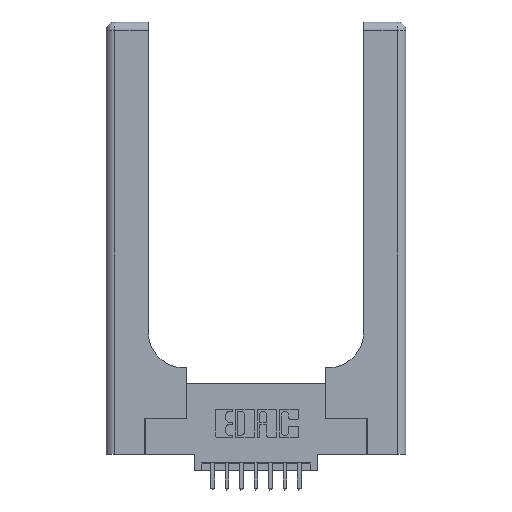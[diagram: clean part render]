
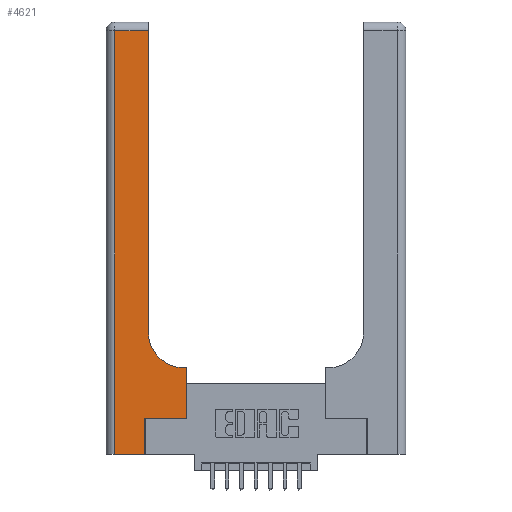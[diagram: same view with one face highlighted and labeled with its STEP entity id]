
A CAD part, top view. The second image highlights one B-rep face of the part: STEP entity #4621.
In plain terms, the highlighted planar face has unit normal (0, 0, 1).
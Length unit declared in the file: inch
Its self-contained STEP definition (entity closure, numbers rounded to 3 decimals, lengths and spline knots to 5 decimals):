
#154 = DIRECTION ( 'NONE',  ( -1., 0., 0. ) ) ;
#246 = CARTESIAN_POINT ( 'NONE',  ( 0., 2.94, 0.37 ) ) ;
#254 = VERTEX_POINT ( 'NONE', #12821 ) ;
#1122 = VERTEX_POINT ( 'NONE', #13491 ) ;
#1332 = LINE ( 'NONE', #9069, #10580 ) ;
#1525 = VECTOR ( 'NONE', #13290, 39.37008 ) ;
#1546 = CARTESIAN_POINT ( 'NONE',  ( 0.06, 3., 0.37 ) ) ;
#1699 = CARTESIAN_POINT ( 'NONE',  ( 0.269, 0.25, 0.37 ) ) ;
#1946 = VERTEX_POINT ( 'NONE', #5998 ) ;
#2030 = DIRECTION ( 'NONE',  ( 0., 0., -1. ) ) ;
#2702 = DIRECTION ( 'NONE',  ( -1., 0., 0. ) ) ;
#2838 = VECTOR ( 'NONE', #15284, 39.37008 ) ;
#3311 = ORIENTED_EDGE ( 'NONE', *, *, #6691, .T. ) ;
#3472 = AXIS2_PLACEMENT_3D ( 'NONE', #9282, #2030, #10478 ) ;
#3573 = ORIENTED_EDGE ( 'NONE', *, *, #14338, .T. ) ;
#3783 = CARTESIAN_POINT ( 'NONE',  ( 0., 3., 0.37 ) ) ;
#3877 = EDGE_CURVE ( 'NONE', #10096, #9780, #14116, .T. ) ;
#4018 = ORIENTED_EDGE ( 'NONE', *, *, #9170, .T. ) ;
#4047 = ORIENTED_EDGE ( 'NONE', *, *, #5280, .T. ) ;
#4137 = EDGE_CURVE ( 'NONE', #1946, #10096, #11156, .T. ) ;
#4266 = ORIENTED_EDGE ( 'NONE', *, *, #7116, .T. ) ;
#4610 = DIRECTION ( 'NONE',  ( 1., 0., 0. ) ) ;
#4621 = ADVANCED_FACE ( 'NONE', ( #14287 ), #9793, .F. ) ;
#5148 = CARTESIAN_POINT ( 'NONE',  ( 0.5415, 0.6, 0.37 ) ) ;
#5280 = EDGE_CURVE ( 'NONE', #13958, #254, #8876, .T. ) ;
#5762 = CARTESIAN_POINT ( 'NONE',  ( 0.5585, 0.6, 0.37 ) ) ;
#5808 = CARTESIAN_POINT ( 'NONE',  ( 0.2915, 3., 0.37 ) ) ;
#5809 = CARTESIAN_POINT ( 'NONE',  ( 0.269, 0.25, 0.37 ) ) ;
#5924 = LINE ( 'NONE', #1546, #15060 ) ;
#5997 = LINE ( 'NONE', #6242, #15127 ) ;
#5998 = CARTESIAN_POINT ( 'NONE',  ( 0.5585, 0.25, 0.37 ) ) ;
#6168 = VERTEX_POINT ( 'NONE', #1699 ) ;
#6242 = CARTESIAN_POINT ( 'NONE',  ( 0., 0., 0.37 ) ) ;
#6462 = VECTOR ( 'NONE', #2702, 39.37008 ) ;
#6691 = EDGE_CURVE ( 'NONE', #7832, #12375, #5997, .T. ) ;
#6827 = ORIENTED_EDGE ( 'NONE', *, *, #10435, .T. ) ;
#7116 = EDGE_CURVE ( 'NONE', #6168, #1946, #15495, .T. ) ;
#7429 = DIRECTION ( 'NONE',  ( 0., 0., -1. ) ) ;
#7473 = DIRECTION ( 'NONE',  ( 1., 0., 0. ) ) ;
#7639 = CARTESIAN_POINT ( 'NONE',  ( 0.269, 0., 0.37 ) ) ;
#7742 = CARTESIAN_POINT ( 'NONE',  ( 0.2915, 0.85, 0.37 ) ) ;
#7799 = VECTOR ( 'NONE', #14010, 39.37008 ) ;
#7832 = VERTEX_POINT ( 'NONE', #13058 ) ;
#8183 = ORIENTED_EDGE ( 'NONE', *, *, #14642, .T. ) ;
#8328 = CIRCLE ( 'NONE', #3472, 0.25 ) ;
#8488 = CARTESIAN_POINT ( 'NONE',  ( 0.5585, 0.25, 0.37 ) ) ;
#8876 = LINE ( 'NONE', #5808, #2838 ) ;
#9069 = CARTESIAN_POINT ( 'NONE',  ( 0.269, 0., 0.37 ) ) ;
#9170 = EDGE_CURVE ( 'NONE', #1122, #7832, #5924, .T. ) ;
#9186 = VECTOR ( 'NONE', #4610, 39.37008 ) ;
#9282 = CARTESIAN_POINT ( 'NONE',  ( 0.5415, 0.85, 0.37 ) ) ;
#9467 = EDGE_LOOP ( 'NONE', ( #4047, #3573, #4018, #3311, #6827, #4266, #12226, #13690, #8183 ) ) ;
#9780 = VERTEX_POINT ( 'NONE', #5148 ) ;
#9793 = PLANE ( 'NONE',  #15289 ) ;
#10096 = VERTEX_POINT ( 'NONE', #5762 ) ;
#10435 = EDGE_CURVE ( 'NONE', #12375, #6168, #1332, .T. ) ;
#10478 = DIRECTION ( 'NONE',  ( 1., 0., 0. ) ) ;
#10580 = VECTOR ( 'NONE', #15026, 39.37008 ) ;
#11148 = DIRECTION ( 'NONE',  ( 0., -1., 0. ) ) ;
#11156 = LINE ( 'NONE', #8488, #1525 ) ;
#11615 = CARTESIAN_POINT ( 'NONE',  ( 0.2915, 0.6, 0.37 ) ) ;
#12226 = ORIENTED_EDGE ( 'NONE', *, *, #4137, .T. ) ;
#12375 = VERTEX_POINT ( 'NONE', #7639 ) ;
#12821 = CARTESIAN_POINT ( 'NONE',  ( 0.2915, 2.94, 0.37 ) ) ;
#13058 = CARTESIAN_POINT ( 'NONE',  ( 0.06, 0., 0.37 ) ) ;
#13290 = DIRECTION ( 'NONE',  ( 0., 1., 0. ) ) ;
#13491 = CARTESIAN_POINT ( 'NONE',  ( 0.06, 2.94, 0.37 ) ) ;
#13690 = ORIENTED_EDGE ( 'NONE', *, *, #3877, .T. ) ;
#13958 = VERTEX_POINT ( 'NONE', #7742 ) ;
#14010 = DIRECTION ( 'NONE',  ( -1., 0., 0. ) ) ;
#14116 = LINE ( 'NONE', #11615, #7799 ) ;
#14287 = FACE_OUTER_BOUND ( 'NONE', #9467, .T. ) ;
#14338 = EDGE_CURVE ( 'NONE', #254, #1122, #15198, .T. ) ;
#14642 = EDGE_CURVE ( 'NONE', #9780, #13958, #8328, .T. ) ;
#15026 = DIRECTION ( 'NONE',  ( 0., 1., 0. ) ) ;
#15060 = VECTOR ( 'NONE', #11148, 39.37008 ) ;
#15127 = VECTOR ( 'NONE', #7473, 39.37008 ) ;
#15198 = LINE ( 'NONE', #246, #6462 ) ;
#15284 = DIRECTION ( 'NONE',  ( 0., 1., 0. ) ) ;
#15289 = AXIS2_PLACEMENT_3D ( 'NONE', #3783, #7429, #154 ) ;
#15495 = LINE ( 'NONE', #5809, #9186 ) ;
